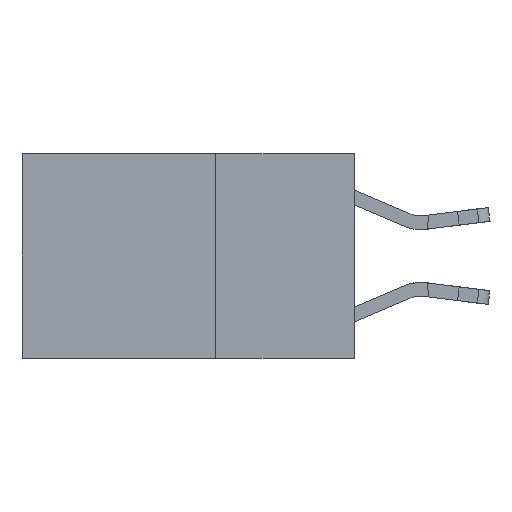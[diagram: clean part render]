
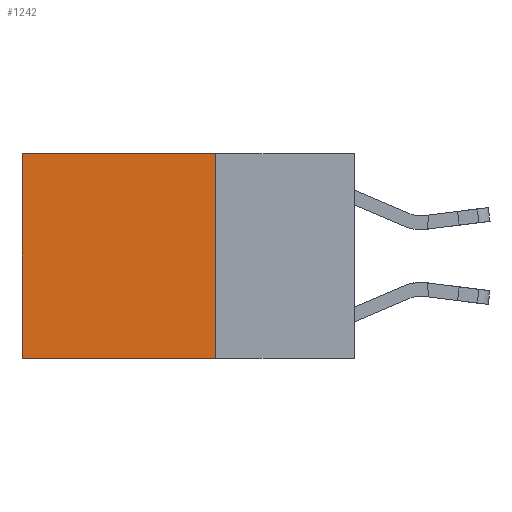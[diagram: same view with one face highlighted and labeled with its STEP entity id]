
A CAD part, left-side view. The second image highlights one B-rep face of the part: STEP entity #1242.
In plain terms, the highlighted planar face has unit normal (-1, 0, 0).
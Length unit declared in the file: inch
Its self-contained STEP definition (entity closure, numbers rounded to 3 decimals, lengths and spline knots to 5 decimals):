
#66 = ORIENTED_EDGE ( 'NONE', *, *, #6839, .F. ) ;
#233 = CARTESIAN_POINT ( 'NONE',  ( 0.2625, 0.6, -0.37 ) ) ;
#1242 = ADVANCED_FACE ( 'NONE', ( #14234 ), #3992, .F. ) ;
#1559 = AXIS2_PLACEMENT_3D ( 'NONE', #22793, #1883, #25018 ) ;
#1883 = DIRECTION ( 'NONE',  ( 1., 0., 0. ) ) ;
#3992 = PLANE ( 'NONE',  #1559 ) ;
#5516 = VECTOR ( 'NONE', #9166, 39.37008 ) ;
#6302 = EDGE_CURVE ( 'NONE', #23345, #7867, #13653, .T. ) ;
#6532 = VECTOR ( 'NONE', #6861, 39.37008 ) ;
#6839 = EDGE_CURVE ( 'NONE', #9153, #23345, #9951, .T. ) ;
#6861 = DIRECTION ( 'NONE',  ( 0., 0., -1. ) ) ;
#6979 = VECTOR ( 'NONE', #15888, 39.37008 ) ;
#7331 = CARTESIAN_POINT ( 'NONE',  ( 0.2625, 0.25, -0.37 ) ) ;
#7867 = VERTEX_POINT ( 'NONE', #233 ) ;
#9153 = VERTEX_POINT ( 'NONE', #12071 ) ;
#9166 = DIRECTION ( 'NONE',  ( 0., 1., 0. ) ) ;
#9951 = LINE ( 'NONE', #20499, #13725 ) ;
#11659 = EDGE_LOOP ( 'NONE', ( #20080, #23511, #66, #25001 ) ) ;
#12071 = CARTESIAN_POINT ( 'NONE',  ( 0.2625, 0.25, 0. ) ) ;
#13653 = LINE ( 'NONE', #7331, #6979 ) ;
#13725 = VECTOR ( 'NONE', #26797, 39.37008 ) ;
#14234 = FACE_OUTER_BOUND ( 'NONE', #11659, .T. ) ;
#15346 = LINE ( 'NONE', #21681, #5516 ) ;
#15888 = DIRECTION ( 'NONE',  ( 0., 1., 0. ) ) ;
#16961 = CARTESIAN_POINT ( 'NONE',  ( 0.2625, 0.6, 0. ) ) ;
#17507 = EDGE_CURVE ( 'NONE', #22839, #7867, #27633, .T. ) ;
#20080 = ORIENTED_EDGE ( 'NONE', *, *, #17507, .T. ) ;
#20499 = CARTESIAN_POINT ( 'NONE',  ( 0.2625, 0.25, 0. ) ) ;
#21681 = CARTESIAN_POINT ( 'NONE',  ( 0.2625, 0.25, 0. ) ) ;
#22793 = CARTESIAN_POINT ( 'NONE',  ( 0.2625, 0.25, 0. ) ) ;
#22839 = VERTEX_POINT ( 'NONE', #16961 ) ;
#23345 = VERTEX_POINT ( 'NONE', #26134 ) ;
#23511 = ORIENTED_EDGE ( 'NONE', *, *, #6302, .F. ) ;
#24774 = EDGE_CURVE ( 'NONE', #9153, #22839, #15346, .T. ) ;
#25001 = ORIENTED_EDGE ( 'NONE', *, *, #24774, .T. ) ;
#25018 = DIRECTION ( 'NONE',  ( 0., 0., -1. ) ) ;
#25530 = CARTESIAN_POINT ( 'NONE',  ( 0.2625, 0.6, 0. ) ) ;
#26134 = CARTESIAN_POINT ( 'NONE',  ( 0.2625, 0.25, -0.37 ) ) ;
#26797 = DIRECTION ( 'NONE',  ( 0., 0., -1. ) ) ;
#27633 = LINE ( 'NONE', #25530, #6532 ) ;
